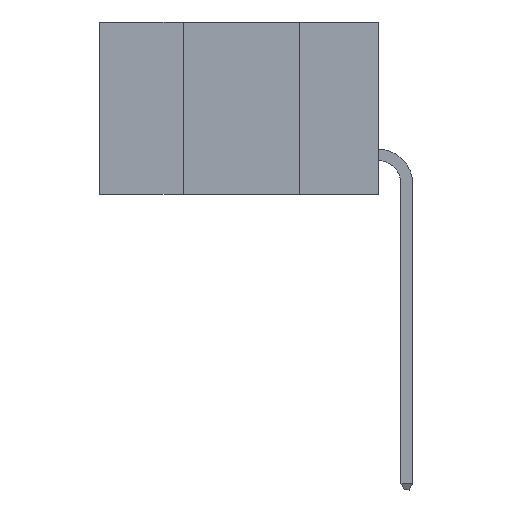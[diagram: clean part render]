
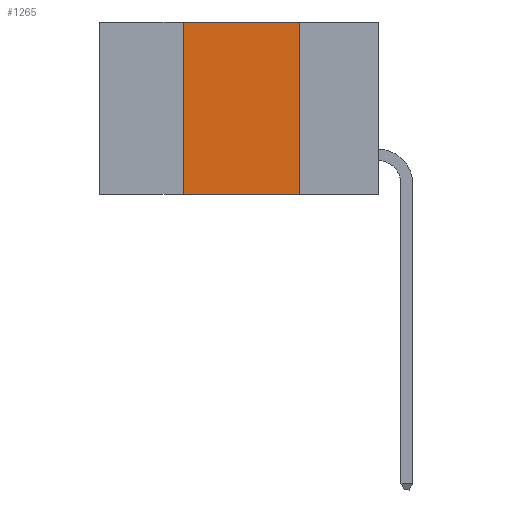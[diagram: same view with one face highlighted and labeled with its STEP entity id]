
A CAD part, left-side view. The second image highlights one B-rep face of the part: STEP entity #1265.
In plain terms, the highlighted planar face has unit normal (-1, 0, 0).
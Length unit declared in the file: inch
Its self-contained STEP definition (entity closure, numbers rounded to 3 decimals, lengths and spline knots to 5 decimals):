
#1265 = ADVANCED_FACE ( 'NONE', ( #9612 ), #22802, .F. ) ;
#1869 = EDGE_CURVE ( 'NONE', #8914, #26703, #18480, .T. ) ;
#2806 = VECTOR ( 'NONE', #15568, 39.37008 ) ;
#3524 = DIRECTION ( 'NONE',  ( 1., 0., 0. ) ) ;
#3932 = LINE ( 'NONE', #8017, #15875 ) ;
#5391 = LINE ( 'NONE', #14029, #28274 ) ;
#7764 = CARTESIAN_POINT ( 'NONE',  ( 0., 0.17, -0.37 ) ) ;
#8017 = CARTESIAN_POINT ( 'NONE',  ( 0., 0.42, 0. ) ) ;
#8755 = ORIENTED_EDGE ( 'NONE', *, *, #14161, .F. ) ;
#8914 = VERTEX_POINT ( 'NONE', #12257 ) ;
#9612 = FACE_OUTER_BOUND ( 'NONE', #11439, .T. ) ;
#10273 = VERTEX_POINT ( 'NONE', #14248 ) ;
#10745 = ORIENTED_EDGE ( 'NONE', *, *, #11309, .F. ) ;
#10942 = LINE ( 'NONE', #26423, #14697 ) ;
#11309 = EDGE_CURVE ( 'NONE', #20846, #8914, #5391, .T. ) ;
#11439 = EDGE_LOOP ( 'NONE', ( #15777, #10745, #8755, #22750 ) ) ;
#12257 = CARTESIAN_POINT ( 'NONE',  ( 0., 0.17, 0. ) ) ;
#13298 = CARTESIAN_POINT ( 'NONE',  ( 0., 0.42, 0. ) ) ;
#14029 = CARTESIAN_POINT ( 'NONE',  ( 0., 0.6, 0. ) ) ;
#14161 = EDGE_CURVE ( 'NONE', #10273, #20846, #3932, .T. ) ;
#14248 = CARTESIAN_POINT ( 'NONE',  ( 0., 0.42, -0.37 ) ) ;
#14603 = DIRECTION ( 'NONE',  ( 0., 0., 1. ) ) ;
#14697 = VECTOR ( 'NONE', #24341, 39.37008 ) ;
#15568 = DIRECTION ( 'NONE',  ( 0., 0., -1. ) ) ;
#15777 = ORIENTED_EDGE ( 'NONE', *, *, #1869, .F. ) ;
#15875 = VECTOR ( 'NONE', #14603, 39.37008 ) ;
#16906 = DIRECTION ( 'NONE',  ( 0., -1., 0. ) ) ;
#17038 = EDGE_CURVE ( 'NONE', #10273, #26703, #10942, .T. ) ;
#18476 = DIRECTION ( 'NONE',  ( 0., 0., -1. ) ) ;
#18480 = LINE ( 'NONE', #22286, #2806 ) ;
#18659 = CARTESIAN_POINT ( 'NONE',  ( 0., 0.6, 0. ) ) ;
#20846 = VERTEX_POINT ( 'NONE', #13298 ) ;
#22286 = CARTESIAN_POINT ( 'NONE',  ( 0., 0.17, 0. ) ) ;
#22750 = ORIENTED_EDGE ( 'NONE', *, *, #17038, .T. ) ;
#22802 = PLANE ( 'NONE',  #23535 ) ;
#23535 = AXIS2_PLACEMENT_3D ( 'NONE', #18659, #3524, #18476 ) ;
#24341 = DIRECTION ( 'NONE',  ( 0., -1., 0. ) ) ;
#26423 = CARTESIAN_POINT ( 'NONE',  ( 0., 0.6, -0.37 ) ) ;
#26703 = VERTEX_POINT ( 'NONE', #7764 ) ;
#28274 = VECTOR ( 'NONE', #16906, 39.37008 ) ;
